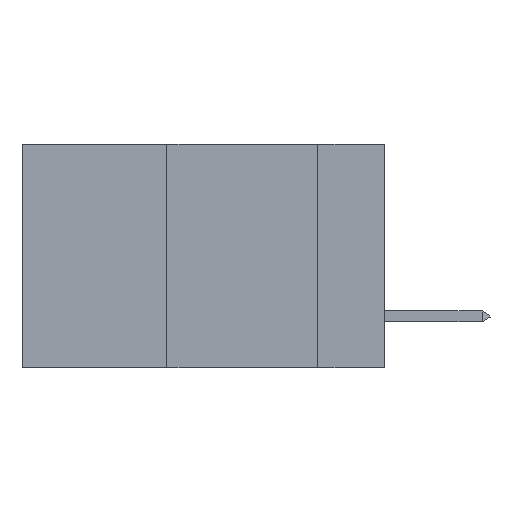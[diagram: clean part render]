
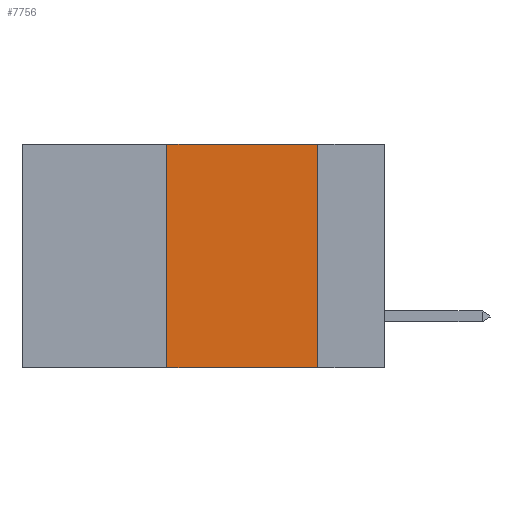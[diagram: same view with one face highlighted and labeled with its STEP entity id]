
A CAD part, left-side view. The second image highlights one B-rep face of the part: STEP entity #7756.
In plain terms, the highlighted planar face has unit normal (-1, 0, 0).
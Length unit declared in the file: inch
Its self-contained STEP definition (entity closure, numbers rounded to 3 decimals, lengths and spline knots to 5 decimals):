
#603 = EDGE_CURVE ( 'NONE', #16258, #27046, #12999, .T. ) ;
#1889 = CARTESIAN_POINT ( 'NONE',  ( 0., 0.11, 0. ) ) ;
#2074 = VECTOR ( 'NONE', #15900, 39.37008 ) ;
#6295 = AXIS2_PLACEMENT_3D ( 'NONE', #15011, #15502, #19466 ) ;
#7756 = ADVANCED_FACE ( 'NONE', ( #30015 ), #29253, .F. ) ;
#8148 = EDGE_CURVE ( 'NONE', #28787, #16258, #19160, .T. ) ;
#9801 = VECTOR ( 'NONE', #18222, 39.37008 ) ;
#10737 = EDGE_LOOP ( 'NONE', ( #22551, #12843, #16336, #25381 ) ) ;
#12081 = CARTESIAN_POINT ( 'NONE',  ( 0., 0.36, 0. ) ) ;
#12843 = ORIENTED_EDGE ( 'NONE', *, *, #8148, .F. ) ;
#12999 = LINE ( 'NONE', #20232, #28870 ) ;
#13026 = VECTOR ( 'NONE', #19384, 39.37008 ) ;
#13322 = LINE ( 'NONE', #22995, #2074 ) ;
#13749 = EDGE_CURVE ( 'NONE', #13843, #28787, #13322, .T. ) ;
#13843 = VERTEX_POINT ( 'NONE', #18655 ) ;
#15011 = CARTESIAN_POINT ( 'NONE',  ( 0., 0.6, 0. ) ) ;
#15102 = CARTESIAN_POINT ( 'NONE',  ( 0., 0.6, 0. ) ) ;
#15502 = DIRECTION ( 'NONE',  ( 1., 0., 0. ) ) ;
#15851 = DIRECTION ( 'NONE',  ( 0., 0., -1. ) ) ;
#15900 = DIRECTION ( 'NONE',  ( 0., 0., 1. ) ) ;
#16258 = VERTEX_POINT ( 'NONE', #1889 ) ;
#16336 = ORIENTED_EDGE ( 'NONE', *, *, #13749, .F. ) ;
#18222 = DIRECTION ( 'NONE',  ( 0., -1., 0. ) ) ;
#18655 = CARTESIAN_POINT ( 'NONE',  ( 0., 0.36, -0.37 ) ) ;
#19160 = LINE ( 'NONE', #15102, #13026 ) ;
#19190 = LINE ( 'NONE', #29603, #9801 ) ;
#19384 = DIRECTION ( 'NONE',  ( 0., -1., 0. ) ) ;
#19466 = DIRECTION ( 'NONE',  ( 0., 0., -1. ) ) ;
#20211 = EDGE_CURVE ( 'NONE', #13843, #27046, #19190, .T. ) ;
#20232 = CARTESIAN_POINT ( 'NONE',  ( 0., 0.11, 0. ) ) ;
#21800 = CARTESIAN_POINT ( 'NONE',  ( 0., 0.11, -0.37 ) ) ;
#22551 = ORIENTED_EDGE ( 'NONE', *, *, #603, .F. ) ;
#22995 = CARTESIAN_POINT ( 'NONE',  ( 0., 0.36, 0. ) ) ;
#25381 = ORIENTED_EDGE ( 'NONE', *, *, #20211, .T. ) ;
#27046 = VERTEX_POINT ( 'NONE', #21800 ) ;
#28787 = VERTEX_POINT ( 'NONE', #12081 ) ;
#28870 = VECTOR ( 'NONE', #15851, 39.37008 ) ;
#29253 = PLANE ( 'NONE',  #6295 ) ;
#29603 = CARTESIAN_POINT ( 'NONE',  ( 0., 0.6, -0.37 ) ) ;
#30015 = FACE_OUTER_BOUND ( 'NONE', #10737, .T. ) ;
